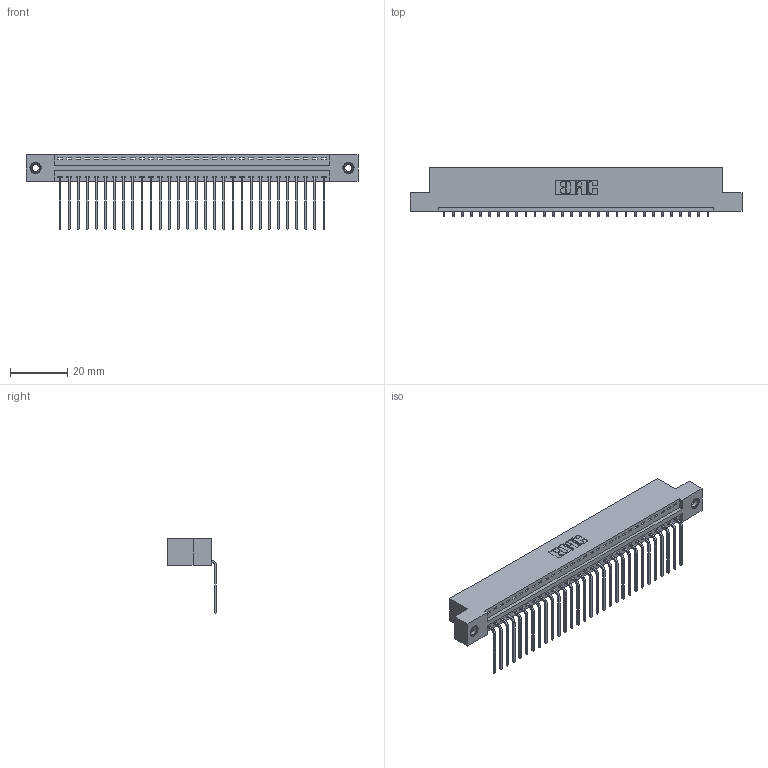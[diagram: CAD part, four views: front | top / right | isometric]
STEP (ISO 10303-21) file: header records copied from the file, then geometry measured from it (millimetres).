
FILE_DESCRIPTION (( 'STEP AP203' ), '1' );
FILE_NAME ('346-030-559-107.STEP', '2022-05-06T16:14:00', ( '' ), ( '' ), 'SwSTEP 2.0', 'SolidWorks 2020', '' );
FILE_SCHEMA (( 'CONFIG_CONTROL_DESIGN' ));
Length unit declared in the file: inch
Products named in the file (4): 346 Part_Flush Mounting Lugs - 0.156 Dia-TI; 345-250-001_345-250-005-103; 346-030-559-107; 345-292-001_558 559 Tail - 1
Assembly tree (33 placements, depth 2):
  346-030-559-107
    346 Part_Flush Mounting Lugs - 0.156 Dia-TI
    345-292-001_558 559 Tail - 1  x30
    345-250-001_345-250-005-103  x2
Bounding box: 115.82 x 17.08 x 26.16 mm (x, y, z)
Volume: 11090.7 mm3; surface area: 14363.4 mm2
Topology: 33 solids, 33 shells, 1982 faces, 5925 edges, 3902 vertices
Faces by surface type: plane 1368, cylinder 598, cone 12, torus 4
Entity records: 21504 total; most frequent: CARTESIAN_POINT 3673, ORIENTED_EDGE 3630, DIRECTION 3281, EDGE_CURVE 1815, VECTOR 1543, LINE 1543, VERTEX_POINT 1204, AXIS2_PLACEMENT_3D 869
